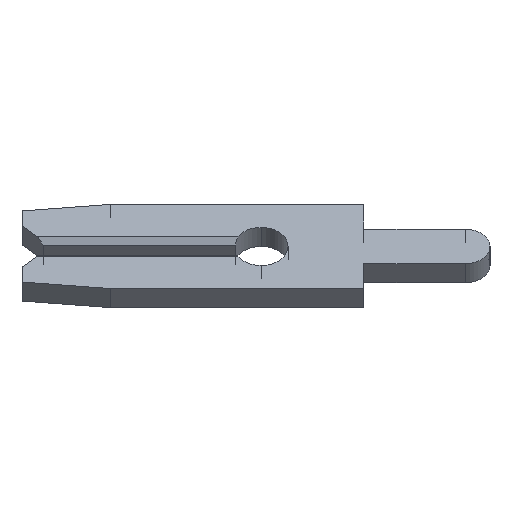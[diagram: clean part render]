
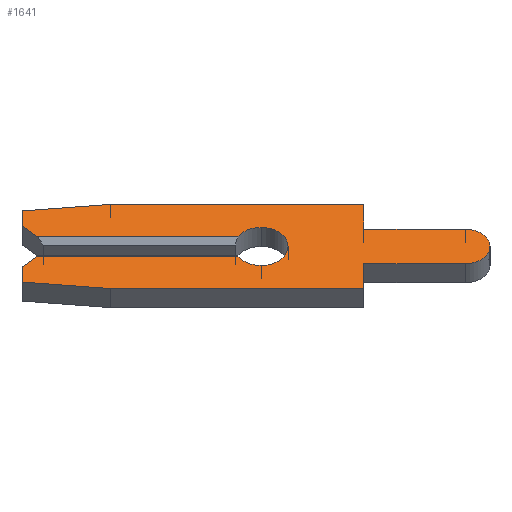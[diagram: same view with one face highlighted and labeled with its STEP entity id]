
A CAD part, left-side view. The second image highlights one B-rep face of the part: STEP entity #1641.
In plain terms, the highlighted face is planar.
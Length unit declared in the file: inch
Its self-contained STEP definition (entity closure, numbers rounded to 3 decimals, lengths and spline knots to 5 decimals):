
#15 = ORIENTED_EDGE ( 'NONE', *, *, #1249, .F. ) ;
#45 = ORIENTED_EDGE ( 'NONE', *, *, #1706, .F. ) ;
#58 = VECTOR ( 'NONE', #925, 39.37008 ) ;
#84 = VECTOR ( 'NONE', #293, 39.37008 ) ;
#89 = DIRECTION ( 'NONE',  ( 0., 1., 0. ) ) ;
#100 = CARTESIAN_POINT ( 'NONE',  ( -0.013, 0.231, -0.028 ) ) ;
#104 = DIRECTION ( 'NONE',  ( 0., 0., 1. ) ) ;
#135 = DIRECTION ( 'NONE',  ( 1., 0., 0. ) ) ;
#145 = PLANE ( 'NONE',  #1047 ) ;
#148 = VERTEX_POINT ( 'NONE', #548 ) ;
#154 = LINE ( 'NONE', #1223, #1636 ) ;
#162 = CARTESIAN_POINT ( 'NONE',  ( -0.013, 0.231, 0.013 ) ) ;
#172 = LINE ( 'NONE', #1516, #1062 ) ;
#177 = CARTESIAN_POINT ( 'NONE',  ( -0.013, 0.146, -0.0575 ) ) ;
#187 = DIRECTION ( 'NONE',  ( 0., -1., 0. ) ) ;
#192 = VERTEX_POINT ( 'NONE', #232 ) ;
#196 = EDGE_CURVE ( 'NONE', #1753, #1554, #788, .T. ) ;
#223 = VECTOR ( 'NONE', #1198, 39.37008 ) ;
#232 = CARTESIAN_POINT ( 'NONE',  ( -0.013, -0.099, 0.0235 ) ) ;
#239 = ORIENTED_EDGE ( 'NONE', *, *, #509, .F. ) ;
#268 = LINE ( 'NONE', #100, #1934 ) ;
#281 = CARTESIAN_POINT ( 'NONE',  ( -0.013, -0.099, 0.0575 ) ) ;
#287 = EDGE_CURVE ( 'NONE', #792, #1890, #1580, .T. ) ;
#293 = DIRECTION ( 'NONE',  ( 0., 0.995, 0.105 ) ) ;
#297 = EDGE_CURVE ( 'NONE', #1843, #1753, #1386, .T. ) ;
#306 = CARTESIAN_POINT ( 'NONE',  ( -0.013, 0., 0. ) ) ;
#311 = DIRECTION ( 'NONE',  ( 0., -1., 0. ) ) ;
#336 = VECTOR ( 'NONE', #906, 39.37008 ) ;
#371 = ORIENTED_EDGE ( 'NONE', *, *, #783, .F. ) ;
#410 = CARTESIAN_POINT ( 'NONE',  ( -0.013, 0., -0.026 ) ) ;
#411 = DIRECTION ( 'NONE',  ( 0., 0., 1. ) ) ;
#444 = CIRCLE ( 'NONE', #1364, 0.026 ) ;
#457 = CARTESIAN_POINT ( 'NONE',  ( -0.013, 0.231, 0.028 ) ) ;
#459 = VERTEX_POINT ( 'NONE', #1355 ) ;
#475 = LINE ( 'NONE', #1416, #58 ) ;
#479 = DIRECTION ( 'NONE',  ( 0., -1., 0. ) ) ;
#502 = ORIENTED_EDGE ( 'NONE', *, *, #287, .F. ) ;
#509 = EDGE_CURVE ( 'NONE', #1311, #658, #268, .T. ) ;
#526 = ORIENTED_EDGE ( 'NONE', *, *, #854, .F. ) ;
#548 = CARTESIAN_POINT ( 'NONE',  ( -0.013, 0.02252, -0.013 ) ) ;
#567 = DIRECTION ( 'NONE',  ( 1., 0., 0. ) ) ;
#572 = FACE_OUTER_BOUND ( 'NONE', #1317, .T. ) ;
#585 = ORIENTED_EDGE ( 'NONE', *, *, #1794, .F. ) ;
#624 = CIRCLE ( 'NONE', #686, 0.026 ) ;
#630 = CARTESIAN_POINT ( 'NONE',  ( -0.013, -0.099, 0.0575 ) ) ;
#655 = EDGE_CURVE ( 'NONE', #792, #1076, #1115, .T. ) ;
#658 = VERTEX_POINT ( 'NONE', #1676 ) ;
#686 = AXIS2_PLACEMENT_3D ( 'NONE', #1897, #1297, #1766 ) ;
#693 = VERTEX_POINT ( 'NONE', #410 ) ;
#694 = VECTOR ( 'NONE', #949, 39.37008 ) ;
#718 = EDGE_CURVE ( 'NONE', #148, #693, #444, .T. ) ;
#722 = CARTESIAN_POINT ( 'NONE',  ( -0.013, 0.2105, 0.0075 ) ) ;
#777 = ORIENTED_EDGE ( 'NONE', *, *, #1666, .F. ) ;
#778 = VERTEX_POINT ( 'NONE', #1661 ) ;
#783 = EDGE_CURVE ( 'NONE', #658, #1987, #172, .T. ) ;
#788 = LINE ( 'NONE', #1025, #1791 ) ;
#792 = VERTEX_POINT ( 'NONE', #1192 ) ;
#854 = EDGE_CURVE ( 'NONE', #1667, #1770, #1648, .T. ) ;
#866 = ORIENTED_EDGE ( 'NONE', *, *, #196, .F. ) ;
#870 = DIRECTION ( 'NONE',  ( 0., -0.707, 0.707 ) ) ;
#878 = CARTESIAN_POINT ( 'NONE',  ( -0.013, 0.02252, 0.013 ) ) ;
#886 = CIRCLE ( 'NONE', #935, 0.026 ) ;
#888 = AXIS2_PLACEMENT_3D ( 'NONE', #1984, #567, #104 ) ;
#906 = DIRECTION ( 'NONE',  ( 0., 0., 1. ) ) ;
#908 = DIRECTION ( 'NONE',  ( 0., 1., 0. ) ) ;
#925 = DIRECTION ( 'NONE',  ( 0., -0.995, 0.105 ) ) ;
#932 = ORIENTED_EDGE ( 'NONE', *, *, #1460, .F. ) ;
#935 = AXIS2_PLACEMENT_3D ( 'NONE', #306, #1711, #1410 ) ;
#937 = CARTESIAN_POINT ( 'NONE',  ( -0.013, -0.1975, 0.0235 ) ) ;
#949 = DIRECTION ( 'NONE',  ( 0., 0., -1. ) ) ;
#975 = CARTESIAN_POINT ( 'NONE',  ( -0.013, -0.099, -0.0575 ) ) ;
#1025 = CARTESIAN_POINT ( 'NONE',  ( -0.013, -0.099, -0.0575 ) ) ;
#1035 = DIRECTION ( 'NONE',  ( 0., -1., 0. ) ) ;
#1047 = AXIS2_PLACEMENT_3D ( 'NONE', #1103, #135, #1401 ) ;
#1062 = VECTOR ( 'NONE', #870, 39.37008 ) ;
#1064 = EDGE_CURVE ( 'NONE', #1814, #1843, #1151, .T. ) ;
#1076 = VERTEX_POINT ( 'NONE', #878 ) ;
#1103 = CARTESIAN_POINT ( 'NONE',  ( -0.013, 0., 0. ) ) ;
#1105 = ORIENTED_EDGE ( 'NONE', *, *, #655, .T. ) ;
#1115 = LINE ( 'NONE', #162, #1432 ) ;
#1121 = ORIENTED_EDGE ( 'NONE', *, *, #1064, .F. ) ;
#1128 = CARTESIAN_POINT ( 'NONE',  ( -0.013, -0.099, 0.0235 ) ) ;
#1151 = CIRCLE ( 'NONE', #888, 0.0235 ) ;
#1161 = VECTOR ( 'NONE', #89, 39.37008 ) ;
#1192 = CARTESIAN_POINT ( 'NONE',  ( -0.013, 0.216, 0.013 ) ) ;
#1198 = DIRECTION ( 'NONE',  ( 0., 0.707, 0.707 ) ) ;
#1216 = ORIENTED_EDGE ( 'NONE', *, *, #1704, .F. ) ;
#1223 = CARTESIAN_POINT ( 'NONE',  ( -0.013, 0., -0.013 ) ) ;
#1225 = CARTESIAN_POINT ( 'NONE',  ( -0.013, 0.231, -0.04857 ) ) ;
#1231 = CARTESIAN_POINT ( 'NONE',  ( -0.013, 0.231, 0.028 ) ) ;
#1249 = EDGE_CURVE ( 'NONE', #1404, #1311, #1754, .T. ) ;
#1253 = EDGE_CURVE ( 'NONE', #1554, #1404, #1705, .T. ) ;
#1297 = DIRECTION ( 'NONE',  ( -1., 0., 0. ) ) ;
#1311 = VERTEX_POINT ( 'NONE', #1225 ) ;
#1317 = EDGE_LOOP ( 'NONE', ( #1105, #932, #777, #1675, #1216, #371, #239, #15, #1712, #866, #1342, #1121, #1457, #1485, #526, #585, #45, #502 ) ) ;
#1320 = LINE ( 'NONE', #1128, #1620 ) ;
#1342 = ORIENTED_EDGE ( 'NONE', *, *, #297, .F. ) ;
#1355 = CARTESIAN_POINT ( 'NONE',  ( -0.013, 0.231, 0.04857 ) ) ;
#1364 = AXIS2_PLACEMENT_3D ( 'NONE', #1816, #1977, #1809 ) ;
#1373 = CARTESIAN_POINT ( 'NONE',  ( -0.013, 0.231, -0.04857 ) ) ;
#1380 = EDGE_CURVE ( 'NONE', #192, #1814, #1320, .T. ) ;
#1386 = LINE ( 'NONE', #1817, #1161 ) ;
#1393 = CARTESIAN_POINT ( 'NONE',  ( -0.013, -0.1975, -0.0235 ) ) ;
#1401 = DIRECTION ( 'NONE',  ( 0., 0., -1. ) ) ;
#1404 = VERTEX_POINT ( 'NONE', #177 ) ;
#1410 = DIRECTION ( 'NONE',  ( 0., 0., -1. ) ) ;
#1416 = CARTESIAN_POINT ( 'NONE',  ( -0.013, 0.231, 0.04857 ) ) ;
#1432 = VECTOR ( 'NONE', #479, 39.37008 ) ;
#1457 = ORIENTED_EDGE ( 'NONE', *, *, #1380, .F. ) ;
#1460 = EDGE_CURVE ( 'NONE', #778, #1076, #624, .T. ) ;
#1485 = ORIENTED_EDGE ( 'NONE', *, *, #1971, .F. ) ;
#1498 = DIRECTION ( 'NONE',  ( 0., 0., -1. ) ) ;
#1516 = CARTESIAN_POINT ( 'NONE',  ( -0.013, 0.2105, -0.0075 ) ) ;
#1554 = VERTEX_POINT ( 'NONE', #975 ) ;
#1563 = CARTESIAN_POINT ( 'NONE',  ( -0.013, 0.146, 0.0575 ) ) ;
#1578 = CARTESIAN_POINT ( 'NONE',  ( -0.013, 0.216, -0.013 ) ) ;
#1580 = LINE ( 'NONE', #722, #223 ) ;
#1587 = VECTOR ( 'NONE', #908, 39.37008 ) ;
#1620 = VECTOR ( 'NONE', #187, 39.37008 ) ;
#1636 = VECTOR ( 'NONE', #311, 39.37008 ) ;
#1641 = ADVANCED_FACE ( 'NONE', ( #572 ), #145, .F. ) ;
#1648 = LINE ( 'NONE', #1967, #1789 ) ;
#1661 = CARTESIAN_POINT ( 'NONE',  ( -0.013, 0., 0.026 ) ) ;
#1666 = EDGE_CURVE ( 'NONE', #693, #778, #886, .T. ) ;
#1667 = VERTEX_POINT ( 'NONE', #1563 ) ;
#1675 = ORIENTED_EDGE ( 'NONE', *, *, #718, .F. ) ;
#1676 = CARTESIAN_POINT ( 'NONE',  ( -0.013, 0.231, -0.028 ) ) ;
#1680 = CARTESIAN_POINT ( 'NONE',  ( -0.013, 0.146, -0.0575 ) ) ;
#1704 = EDGE_CURVE ( 'NONE', #1987, #148, #154, .T. ) ;
#1705 = LINE ( 'NONE', #1680, #1587 ) ;
#1706 = EDGE_CURVE ( 'NONE', #1890, #459, #1779, .T. ) ;
#1711 = DIRECTION ( 'NONE',  ( -1., 0., 0. ) ) ;
#1712 = ORIENTED_EDGE ( 'NONE', *, *, #1253, .F. ) ;
#1722 = CARTESIAN_POINT ( 'NONE',  ( -0.013, -0.099, -0.0235 ) ) ;
#1753 = VERTEX_POINT ( 'NONE', #1722 ) ;
#1754 = LINE ( 'NONE', #1373, #84 ) ;
#1766 = DIRECTION ( 'NONE',  ( 0., 0., -1. ) ) ;
#1770 = VERTEX_POINT ( 'NONE', #281 ) ;
#1779 = LINE ( 'NONE', #457, #336 ) ;
#1789 = VECTOR ( 'NONE', #1035, 39.37008 ) ;
#1791 = VECTOR ( 'NONE', #1498, 39.37008 ) ;
#1794 = EDGE_CURVE ( 'NONE', #459, #1667, #475, .T. ) ;
#1809 = DIRECTION ( 'NONE',  ( 0., 0., -1. ) ) ;
#1814 = VERTEX_POINT ( 'NONE', #937 ) ;
#1816 = CARTESIAN_POINT ( 'NONE',  ( -0.013, 0., 0. ) ) ;
#1817 = CARTESIAN_POINT ( 'NONE',  ( -0.013, -0.099, -0.0235 ) ) ;
#1843 = VERTEX_POINT ( 'NONE', #1393 ) ;
#1890 = VERTEX_POINT ( 'NONE', #1231 ) ;
#1894 = LINE ( 'NONE', #630, #694 ) ;
#1897 = CARTESIAN_POINT ( 'NONE',  ( -0.013, 0., 0. ) ) ;
#1934 = VECTOR ( 'NONE', #411, 39.37008 ) ;
#1967 = CARTESIAN_POINT ( 'NONE',  ( -0.013, 0.146, 0.0575 ) ) ;
#1971 = EDGE_CURVE ( 'NONE', #1770, #192, #1894, .T. ) ;
#1977 = DIRECTION ( 'NONE',  ( -1., 0., 0. ) ) ;
#1984 = CARTESIAN_POINT ( 'NONE',  ( -0.013, -0.1975, 0. ) ) ;
#1987 = VERTEX_POINT ( 'NONE', #1578 ) ;
